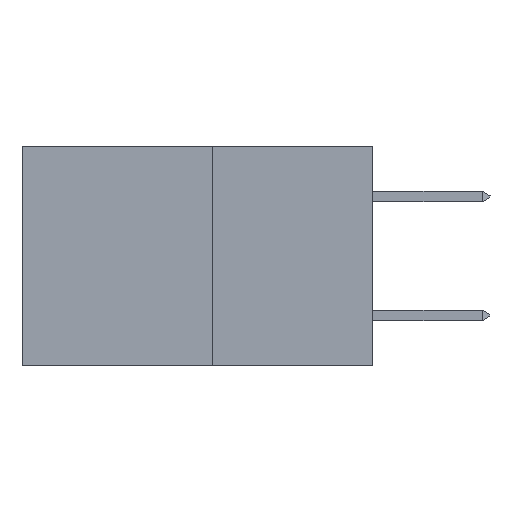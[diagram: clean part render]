
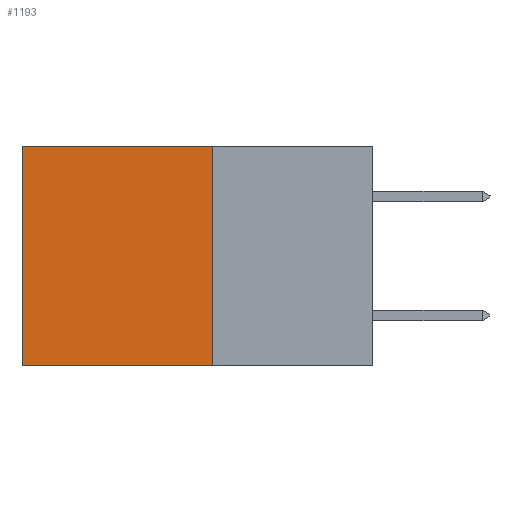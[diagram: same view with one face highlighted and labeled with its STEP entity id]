
A CAD part, left-side view. The second image highlights one B-rep face of the part: STEP entity #1193.
In plain terms, the highlighted planar face has unit normal (-1, 0, 0).
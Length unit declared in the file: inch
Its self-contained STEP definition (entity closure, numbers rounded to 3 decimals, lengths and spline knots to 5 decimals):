
#513 = VECTOR ( 'NONE', #4887, 39.37008 ) ;
#597 = EDGE_CURVE ( 'NONE', #2303, #1521, #17615, .T. ) ;
#855 = ORIENTED_EDGE ( 'NONE', *, *, #20310, .F. ) ;
#1193 = ADVANCED_FACE ( 'NONE', ( #11026 ), #5236, .F. ) ;
#1521 = VERTEX_POINT ( 'NONE', #2306 ) ;
#1886 = ORIENTED_EDGE ( 'NONE', *, *, #17480, .T. ) ;
#2303 = VERTEX_POINT ( 'NONE', #19135 ) ;
#2306 = CARTESIAN_POINT ( 'NONE',  ( 0.277, 0.59, -0.37 ) ) ;
#3240 = CARTESIAN_POINT ( 'NONE',  ( 0.277, 0.27, -0.37 ) ) ;
#3506 = ORIENTED_EDGE ( 'NONE', *, *, #9126, .F. ) ;
#4887 = DIRECTION ( 'NONE',  ( 0., 0., -1. ) ) ;
#5100 = DIRECTION ( 'NONE',  ( 0., 0., -1. ) ) ;
#5105 = DIRECTION ( 'NONE',  ( 1., 0., 0. ) ) ;
#5197 = CARTESIAN_POINT ( 'NONE',  ( 0.277, 0.27, -0.37 ) ) ;
#5236 = PLANE ( 'NONE',  #17525 ) ;
#5427 = ORIENTED_EDGE ( 'NONE', *, *, #597, .T. ) ;
#5572 = VECTOR ( 'NONE', #9858, 39.37008 ) ;
#7839 = VECTOR ( 'NONE', #19754, 39.37008 ) ;
#8158 = VERTEX_POINT ( 'NONE', #18452 ) ;
#9126 = EDGE_CURVE ( 'NONE', #20503, #1521, #12582, .T. ) ;
#9835 = CARTESIAN_POINT ( 'NONE',  ( 0.277, 0.59, -0.37 ) ) ;
#9858 = DIRECTION ( 'NONE',  ( 0., 0., -1. ) ) ;
#10863 = CARTESIAN_POINT ( 'NONE',  ( 0.277, 0.27, -0.37 ) ) ;
#11026 = FACE_OUTER_BOUND ( 'NONE', #15876, .T. ) ;
#12582 = LINE ( 'NONE', #10863, #7839 ) ;
#13412 = CARTESIAN_POINT ( 'NONE',  ( 0.277, 0.27, -0.37 ) ) ;
#13514 = CARTESIAN_POINT ( 'NONE',  ( 0.277, 0.27, 0. ) ) ;
#14851 = LINE ( 'NONE', #13514, #19734 ) ;
#15052 = DIRECTION ( 'NONE',  ( 0., 1., 0. ) ) ;
#15876 = EDGE_LOOP ( 'NONE', ( #5427, #3506, #855, #1886 ) ) ;
#17480 = EDGE_CURVE ( 'NONE', #8158, #2303, #14851, .T. ) ;
#17525 = AXIS2_PLACEMENT_3D ( 'NONE', #5197, #5105, #5100 ) ;
#17615 = LINE ( 'NONE', #9835, #5572 ) ;
#18038 = LINE ( 'NONE', #3240, #513 ) ;
#18452 = CARTESIAN_POINT ( 'NONE',  ( 0.277, 0.27, 0. ) ) ;
#19135 = CARTESIAN_POINT ( 'NONE',  ( 0.277, 0.59, 0. ) ) ;
#19734 = VECTOR ( 'NONE', #15052, 39.37008 ) ;
#19754 = DIRECTION ( 'NONE',  ( 0., 1., 0. ) ) ;
#20310 = EDGE_CURVE ( 'NONE', #8158, #20503, #18038, .T. ) ;
#20503 = VERTEX_POINT ( 'NONE', #13412 ) ;
